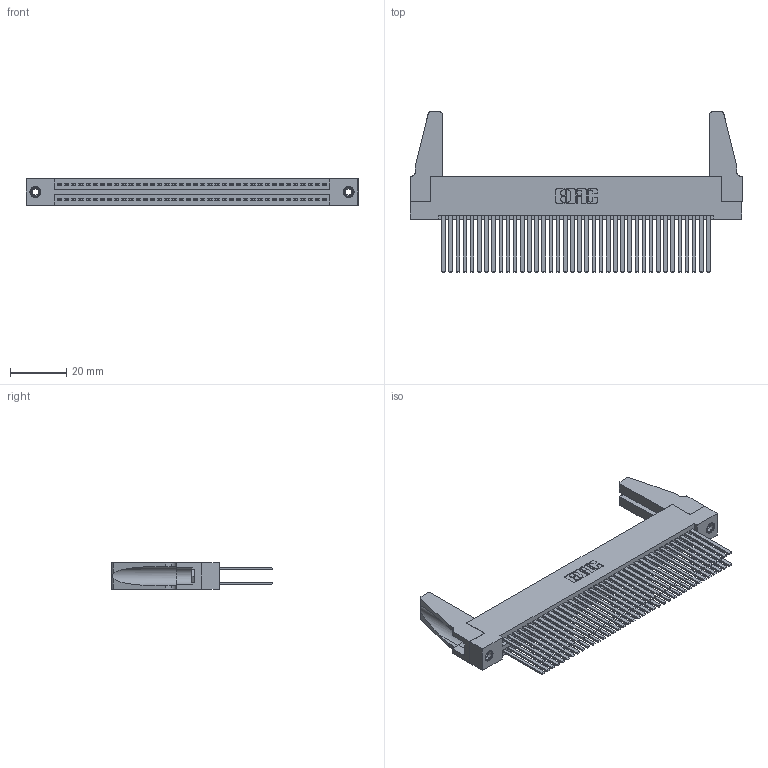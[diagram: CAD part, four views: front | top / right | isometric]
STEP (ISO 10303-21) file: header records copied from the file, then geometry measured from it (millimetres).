
FILE_DESCRIPTION (( 'STEP AP203' ), '1' );
FILE_NAME ('345-076-544-288.STEP', '2019-10-31T13:06:34', ( '' ), ( '' ), 'SwSTEP 2.0', 'SolidWorks 2016', '' );
FILE_SCHEMA (( 'CONFIG_CONTROL_DESIGN' ));
Length unit declared in the file: inch
Products named in the file (5): 345-220-078_345-220-088; 345-250-001_345-250-001-102; 345-076-544-288; 345-292-001_345-293-144; 345 Part_Flush Mounting Lugs - 0.156 Dia-TH
Assembly tree (81 placements, depth 2):
  345-076-544-288
    345 Part_Flush Mounting Lugs - 0.156 Dia-TH
    345-292-001_345-293-144  x76
    345-250-001_345-250-001-102  x2
    345-220-078_345-220-088  x2
Bounding box: 117.75 x 56.82 x 9.4 mm (x, y, z)
Volume: 15719.5 mm3; surface area: 24595.6 mm2
Topology: 81 solids, 81 shells, 3594 faces, 10611 edges, 6962 vertices
Faces by surface type: plane 2356, cylinder 1222, cone 12, torus 4
Entity records: 32318 total; most frequent: CARTESIAN_POINT 5414, ORIENTED_EDGE 5308, DIRECTION 4782, EDGE_CURVE 2654, LINE 2332, VECTOR 2332, VERTEX_POINT 1762, AXIS2_PLACEMENT_3D 1225
